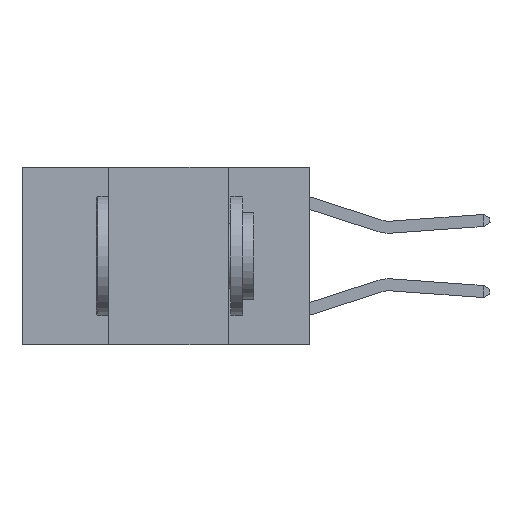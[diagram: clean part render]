
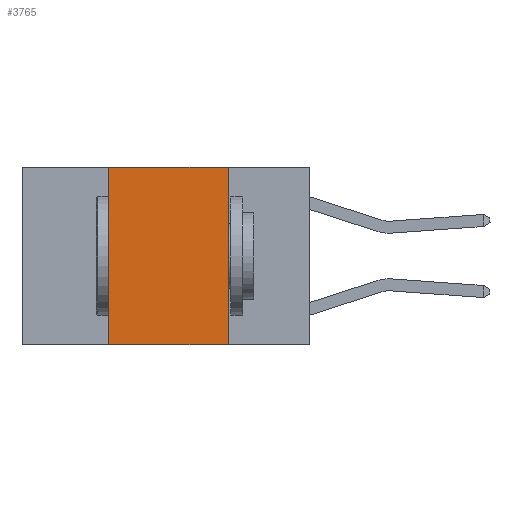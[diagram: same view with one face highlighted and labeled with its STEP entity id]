
A CAD part, left-side view. The second image highlights one B-rep face of the part: STEP entity #3765.
In plain terms, the highlighted planar face has unit normal (-1, 0, 0).
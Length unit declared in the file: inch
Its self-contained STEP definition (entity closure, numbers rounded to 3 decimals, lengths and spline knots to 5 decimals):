
#58 = AXIS2_PLACEMENT_3D ( 'NONE', #8605, #14382, #10072 ) ;
#1160 = VECTOR ( 'NONE', #6894, 39.37008 ) ;
#1813 = DIRECTION ( 'NONE',  ( 0., 0., -1. ) ) ;
#2093 = DIRECTION ( 'NONE',  ( 0., -1., 0. ) ) ;
#2519 = ORIENTED_EDGE ( 'NONE', *, *, #4436, .F. ) ;
#2884 = DIRECTION ( 'NONE',  ( 0., -1., 0. ) ) ;
#3765 = ADVANCED_FACE ( 'NONE', ( #11425 ), #17226, .F. ) ;
#4013 = EDGE_CURVE ( 'NONE', #15411, #18843, #7716, .T. ) ;
#4436 = EDGE_CURVE ( 'NONE', #15411, #16897, #15946, .T. ) ;
#4832 = CARTESIAN_POINT ( 'NONE',  ( 0., 0.17, 0. ) ) ;
#4935 = VECTOR ( 'NONE', #1813, 39.37008 ) ;
#6480 = EDGE_CURVE ( 'NONE', #16897, #12290, #6571, .T. ) ;
#6571 = LINE ( 'NONE', #12099, #10601 ) ;
#6730 = VECTOR ( 'NONE', #2093, 39.37008 ) ;
#6894 = DIRECTION ( 'NONE',  ( 0., 0., 1. ) ) ;
#7716 = LINE ( 'NONE', #15785, #6730 ) ;
#8605 = CARTESIAN_POINT ( 'NONE',  ( 0., 0.6, 0. ) ) ;
#9096 = LINE ( 'NONE', #15474, #4935 ) ;
#10072 = DIRECTION ( 'NONE',  ( 0., 0., -1. ) ) ;
#10108 = CARTESIAN_POINT ( 'NONE',  ( 0., 0.42, -0.37 ) ) ;
#10601 = VECTOR ( 'NONE', #2884, 39.37008 ) ;
#11342 = CARTESIAN_POINT ( 'NONE',  ( 0., 0.42, 0. ) ) ;
#11425 = FACE_OUTER_BOUND ( 'NONE', #17283, .T. ) ;
#11588 = EDGE_CURVE ( 'NONE', #12290, #18843, #9096, .T. ) ;
#12099 = CARTESIAN_POINT ( 'NONE',  ( 0., 0.6, 0. ) ) ;
#12290 = VERTEX_POINT ( 'NONE', #4832 ) ;
#14351 = CARTESIAN_POINT ( 'NONE',  ( 0., 0.17, -0.37 ) ) ;
#14382 = DIRECTION ( 'NONE',  ( 1., 0., 0. ) ) ;
#15411 = VERTEX_POINT ( 'NONE', #10108 ) ;
#15474 = CARTESIAN_POINT ( 'NONE',  ( 0., 0.17, 0. ) ) ;
#15699 = CARTESIAN_POINT ( 'NONE',  ( 0., 0.42, 0. ) ) ;
#15785 = CARTESIAN_POINT ( 'NONE',  ( 0., 0.6, -0.37 ) ) ;
#15946 = LINE ( 'NONE', #15699, #1160 ) ;
#16257 = ORIENTED_EDGE ( 'NONE', *, *, #4013, .T. ) ;
#16897 = VERTEX_POINT ( 'NONE', #11342 ) ;
#17226 = PLANE ( 'NONE',  #58 ) ;
#17283 = EDGE_LOOP ( 'NONE', ( #19245, #17966, #2519, #16257 ) ) ;
#17966 = ORIENTED_EDGE ( 'NONE', *, *, #6480, .F. ) ;
#18843 = VERTEX_POINT ( 'NONE', #14351 ) ;
#19245 = ORIENTED_EDGE ( 'NONE', *, *, #11588, .F. ) ;
